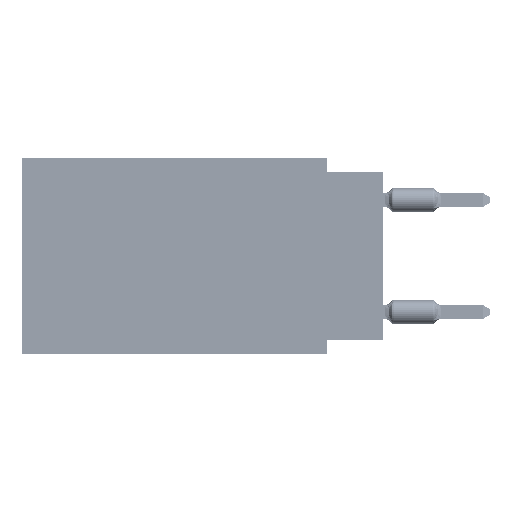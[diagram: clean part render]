
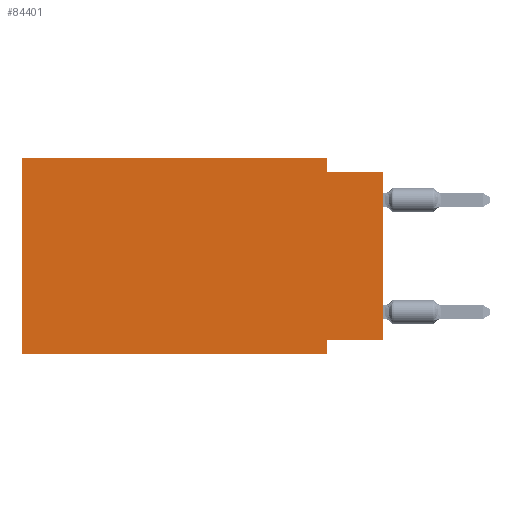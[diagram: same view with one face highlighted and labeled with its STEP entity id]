
A CAD part, left-side view. The second image highlights one B-rep face of the part: STEP entity #84401.
In plain terms, the highlighted planar face has unit normal (-1, 0, 0).
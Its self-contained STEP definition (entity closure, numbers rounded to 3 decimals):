
#1573 = EDGE_CURVE ( 'NONE', #44207, #2424, #54674, .T. ) ;
#1730 = CARTESIAN_POINT ( 'NONE',  ( 0., 2.54, 0. ) ) ;
#1919 = LINE ( 'NONE', #54779, #30107 ) ;
#2424 = VERTEX_POINT ( 'NONE', #62395 ) ;
#2879 = VECTOR ( 'NONE', #53594, 1000. ) ;
#4268 = VECTOR ( 'NONE', #92800, 1000. ) ;
#7663 = VECTOR ( 'NONE', #89985, 1000. ) ;
#8416 = ORIENTED_EDGE ( 'NONE', *, *, #51066, .T. ) ;
#13062 = EDGE_LOOP ( 'NONE', ( #90898, #14282, #43876, #59513, #34281, #8416, #29217, #31685 ) ) ;
#13950 = LINE ( 'NONE', #15430, #38049 ) ;
#14282 = ORIENTED_EDGE ( 'NONE', *, *, #78358, .F. ) ;
#14943 = DIRECTION ( 'NONE',  ( 0., -1., 0. ) ) ;
#15430 = CARTESIAN_POINT ( 'NONE',  ( 0., 16.383, 0. ) ) ;
#16922 = VERTEX_POINT ( 'NONE', #62527 ) ;
#19530 = DIRECTION ( 'NONE',  ( 1., 0., 0. ) ) ;
#21568 = VECTOR ( 'NONE', #77037, 1000. ) ;
#22407 = DIRECTION ( 'NONE',  ( 0., -1., 0. ) ) ;
#24284 = DIRECTION ( 'NONE',  ( 0., 0., 1. ) ) ;
#25198 = VERTEX_POINT ( 'NONE', #84118 ) ;
#29217 = ORIENTED_EDGE ( 'NONE', *, *, #51082, .F. ) ;
#30107 = VECTOR ( 'NONE', #22407, 1000. ) ;
#30998 = EDGE_CURVE ( 'NONE', #69519, #25198, #69537, .T. ) ;
#31162 = LINE ( 'NONE', #91482, #2879 ) ;
#31428 = CARTESIAN_POINT ( 'NONE',  ( 0., 16.383, -8.89 ) ) ;
#31685 = ORIENTED_EDGE ( 'NONE', *, *, #42613, .F. ) ;
#31997 = LINE ( 'NONE', #40936, #4268 ) ;
#33979 = PLANE ( 'NONE',  #84764 ) ;
#34281 = ORIENTED_EDGE ( 'NONE', *, *, #66223, .F. ) ;
#38049 = VECTOR ( 'NONE', #14943, 1000. ) ;
#38265 = CARTESIAN_POINT ( 'NONE',  ( 0., 2.54, -8.255 ) ) ;
#39079 = VERTEX_POINT ( 'NONE', #90059 ) ;
#40075 = DIRECTION ( 'NONE',  ( 0., 0., 1. ) ) ;
#40936 = CARTESIAN_POINT ( 'NONE',  ( 0., 0., -8.255 ) ) ;
#41464 = FACE_OUTER_BOUND ( 'NONE', #13062, .T. ) ;
#42613 = EDGE_CURVE ( 'NONE', #44207, #49321, #31997, .T. ) ;
#43876 = ORIENTED_EDGE ( 'NONE', *, *, #30998, .F. ) ;
#44207 = VERTEX_POINT ( 'NONE', #69728 ) ;
#46146 = CARTESIAN_POINT ( 'NONE',  ( 0., 2.54, 0. ) ) ;
#49321 = VERTEX_POINT ( 'NONE', #38265 ) ;
#51066 = EDGE_CURVE ( 'NONE', #98355, #39079, #31162, .T. ) ;
#51082 = EDGE_CURVE ( 'NONE', #49321, #39079, #61566, .T. ) ;
#51741 = EDGE_CURVE ( 'NONE', #16922, #69519, #13950, .T. ) ;
#53594 = DIRECTION ( 'NONE',  ( 0., -1., 0. ) ) ;
#54674 = LINE ( 'NONE', #62149, #66008 ) ;
#54779 = CARTESIAN_POINT ( 'NONE',  ( 0., 0., -0.635 ) ) ;
#59513 = ORIENTED_EDGE ( 'NONE', *, *, #51741, .F. ) ;
#60766 = VECTOR ( 'NONE', #40075, 1000. ) ;
#61566 = LINE ( 'NONE', #83520, #7663 ) ;
#62004 = CARTESIAN_POINT ( 'NONE',  ( 0., 16.383, 0. ) ) ;
#62149 = CARTESIAN_POINT ( 'NONE',  ( 0., 0., 0. ) ) ;
#62395 = CARTESIAN_POINT ( 'NONE',  ( 0., 0., -0.635 ) ) ;
#62527 = CARTESIAN_POINT ( 'NONE',  ( 0., 16.383, 0. ) ) ;
#64364 = CARTESIAN_POINT ( 'NONE',  ( 0., 16.383, 0. ) ) ;
#66008 = VECTOR ( 'NONE', #24284, 1000. ) ;
#66223 = EDGE_CURVE ( 'NONE', #98355, #16922, #92896, .T. ) ;
#69519 = VERTEX_POINT ( 'NONE', #46146 ) ;
#69537 = LINE ( 'NONE', #1730, #21568 ) ;
#69728 = CARTESIAN_POINT ( 'NONE',  ( 0., 0., -8.255 ) ) ;
#77037 = DIRECTION ( 'NONE',  ( 0., 0., -1. ) ) ;
#78358 = EDGE_CURVE ( 'NONE', #25198, #2424, #1919, .T. ) ;
#83520 = CARTESIAN_POINT ( 'NONE',  ( 0., 2.54, -8.89 ) ) ;
#84118 = CARTESIAN_POINT ( 'NONE',  ( 0., 2.54, -0.635 ) ) ;
#84401 = ADVANCED_FACE ( 'NONE', ( #41464 ), #33979, .F. ) ;
#84764 = AXIS2_PLACEMENT_3D ( 'NONE', #64364, #19530, #94768 ) ;
#89985 = DIRECTION ( 'NONE',  ( 0., 0., -1. ) ) ;
#90059 = CARTESIAN_POINT ( 'NONE',  ( 0., 2.54, -8.89 ) ) ;
#90898 = ORIENTED_EDGE ( 'NONE', *, *, #1573, .T. ) ;
#91482 = CARTESIAN_POINT ( 'NONE',  ( 0., 16.383, -8.89 ) ) ;
#92800 = DIRECTION ( 'NONE',  ( 0., 1., 0. ) ) ;
#92896 = LINE ( 'NONE', #62004, #60766 ) ;
#94768 = DIRECTION ( 'NONE',  ( 0., 0., -1. ) ) ;
#98355 = VERTEX_POINT ( 'NONE', #31428 ) ;
